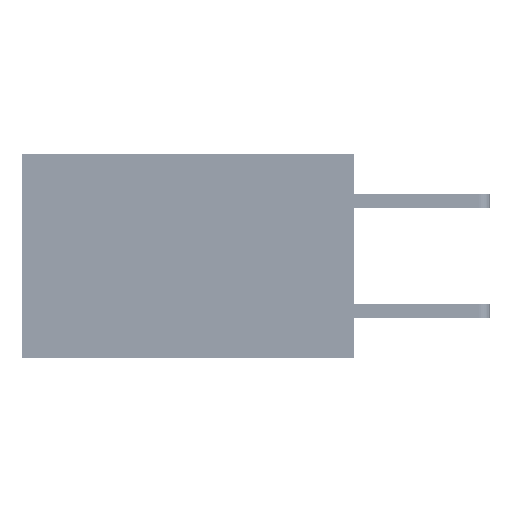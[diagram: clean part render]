
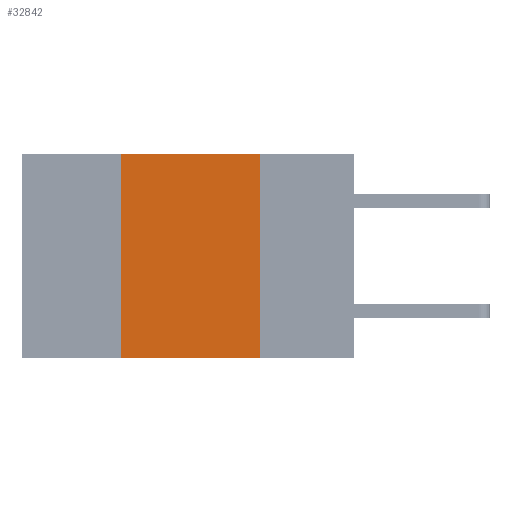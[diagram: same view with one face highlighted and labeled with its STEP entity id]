
A CAD part, left-side view. The second image highlights one B-rep face of the part: STEP entity #32842.
In plain terms, the highlighted planar face has unit normal (-1, 0, 0).
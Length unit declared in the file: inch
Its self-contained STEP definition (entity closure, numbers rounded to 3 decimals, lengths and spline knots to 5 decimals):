
#757 = CARTESIAN_POINT ( 'NONE',  ( 0., 0.6, 0. ) ) ;
#6639 = VECTOR ( 'NONE', #27119, 39.37008 ) ;
#7585 = CARTESIAN_POINT ( 'NONE',  ( 0., 0.42, 0. ) ) ;
#7718 = CARTESIAN_POINT ( 'NONE',  ( 0., 0.17, 0. ) ) ;
#11365 = CARTESIAN_POINT ( 'NONE',  ( 0., 0.42, 0. ) ) ;
#11729 = VERTEX_POINT ( 'NONE', #13507 ) ;
#12014 = LINE ( 'NONE', #7718, #39001 ) ;
#12932 = EDGE_CURVE ( 'NONE', #52197, #11729, #12014, .T. ) ;
#13507 = CARTESIAN_POINT ( 'NONE',  ( 0., 0.17, -0.37 ) ) ;
#16167 = DIRECTION ( 'NONE',  ( 1., 0., 0. ) ) ;
#17148 = DIRECTION ( 'NONE',  ( 0., -1., 0. ) ) ;
#17311 = EDGE_LOOP ( 'NONE', ( #33809, #43054, #25773, #33834 ) ) ;
#23422 = DIRECTION ( 'NONE',  ( 0., 0., -1. ) ) ;
#24065 = VECTOR ( 'NONE', #48359, 39.37008 ) ;
#24340 = DIRECTION ( 'NONE',  ( 0., 0., -1. ) ) ;
#25773 = ORIENTED_EDGE ( 'NONE', *, *, #27485, .F. ) ;
#26716 = CARTESIAN_POINT ( 'NONE',  ( 0., 0.17, 0. ) ) ;
#26876 = AXIS2_PLACEMENT_3D ( 'NONE', #43773, #16167, #23422 ) ;
#27119 = DIRECTION ( 'NONE',  ( 0., -1., 0. ) ) ;
#27485 = EDGE_CURVE ( 'NONE', #46193, #46454, #52366, .T. ) ;
#28856 = EDGE_CURVE ( 'NONE', #46454, #52197, #37500, .T. ) ;
#31920 = CARTESIAN_POINT ( 'NONE',  ( 0., 0.6, -0.37 ) ) ;
#32842 = ADVANCED_FACE ( 'NONE', ( #48086 ), #52881, .F. ) ;
#33809 = ORIENTED_EDGE ( 'NONE', *, *, #12932, .F. ) ;
#33834 = ORIENTED_EDGE ( 'NONE', *, *, #46943, .T. ) ;
#37500 = LINE ( 'NONE', #757, #42105 ) ;
#39001 = VECTOR ( 'NONE', #24340, 39.37008 ) ;
#42105 = VECTOR ( 'NONE', #17148, 39.37008 ) ;
#43054 = ORIENTED_EDGE ( 'NONE', *, *, #28856, .F. ) ;
#43773 = CARTESIAN_POINT ( 'NONE',  ( 0., 0.6, 0. ) ) ;
#45419 = CARTESIAN_POINT ( 'NONE',  ( 0., 0.42, -0.37 ) ) ;
#46193 = VERTEX_POINT ( 'NONE', #45419 ) ;
#46454 = VERTEX_POINT ( 'NONE', #7585 ) ;
#46943 = EDGE_CURVE ( 'NONE', #46193, #11729, #52274, .T. ) ;
#48086 = FACE_OUTER_BOUND ( 'NONE', #17311, .T. ) ;
#48359 = DIRECTION ( 'NONE',  ( 0., 0., 1. ) ) ;
#52197 = VERTEX_POINT ( 'NONE', #26716 ) ;
#52274 = LINE ( 'NONE', #31920, #6639 ) ;
#52366 = LINE ( 'NONE', #11365, #24065 ) ;
#52881 = PLANE ( 'NONE',  #26876 ) ;
